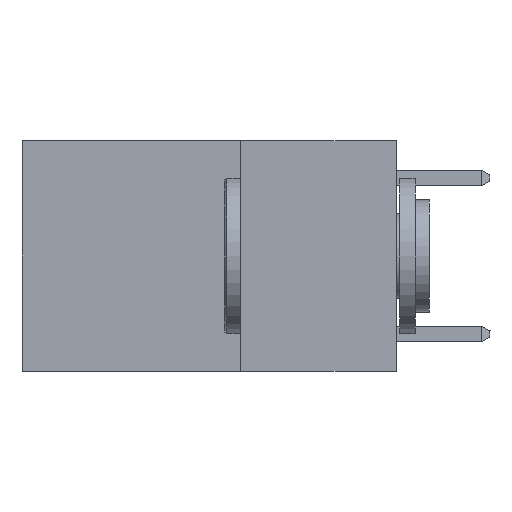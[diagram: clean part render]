
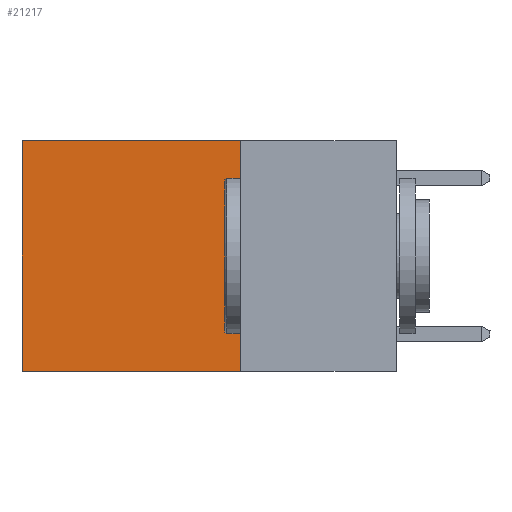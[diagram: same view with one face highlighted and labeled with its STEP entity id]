
A CAD part, left-side view. The second image highlights one B-rep face of the part: STEP entity #21217.
In plain terms, the highlighted planar face has unit normal (-1, 0, 0).
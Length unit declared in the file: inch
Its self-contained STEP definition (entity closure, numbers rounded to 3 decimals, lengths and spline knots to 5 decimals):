
#275 = CARTESIAN_POINT ( 'NONE',  ( 0.2625, 0.6, 0. ) ) ;
#626 = LINE ( 'NONE', #275, #7732 ) ;
#3592 = ORIENTED_EDGE ( 'NONE', *, *, #16844, .T. ) ;
#4262 = CARTESIAN_POINT ( 'NONE',  ( 0.2625, 0.25, -0.37 ) ) ;
#5651 = AXIS2_PLACEMENT_3D ( 'NONE', #19839, #7874, #24626 ) ;
#5946 = CARTESIAN_POINT ( 'NONE',  ( 0.2625, 0.25, 0. ) ) ;
#6872 = CARTESIAN_POINT ( 'NONE',  ( 0.2625, 0.25, -0.37 ) ) ;
#7732 = VECTOR ( 'NONE', #24258, 39.37008 ) ;
#7874 = DIRECTION ( 'NONE',  ( 1., 0., 0. ) ) ;
#11036 = FACE_OUTER_BOUND ( 'NONE', #11213, .T. ) ;
#11213 = EDGE_LOOP ( 'NONE', ( #16848, #19239, #18117, #3592 ) ) ;
#11928 = EDGE_CURVE ( 'NONE', #29138, #14892, #626, .T. ) ;
#12574 = PLANE ( 'NONE',  #5651 ) ;
#13385 = LINE ( 'NONE', #4262, #14127 ) ;
#13697 = EDGE_CURVE ( 'NONE', #24052, #15605, #14722, .T. ) ;
#14127 = VECTOR ( 'NONE', #21028, 39.37008 ) ;
#14722 = LINE ( 'NONE', #27965, #20397 ) ;
#14892 = VERTEX_POINT ( 'NONE', #18669 ) ;
#15488 = CARTESIAN_POINT ( 'NONE',  ( 0.2625, 0.6, 0. ) ) ;
#15605 = VERTEX_POINT ( 'NONE', #6872 ) ;
#15708 = CARTESIAN_POINT ( 'NONE',  ( 0.2625, 0.25, 0. ) ) ;
#16844 = EDGE_CURVE ( 'NONE', #24052, #29138, #19547, .T. ) ;
#16848 = ORIENTED_EDGE ( 'NONE', *, *, #11928, .T. ) ;
#18117 = ORIENTED_EDGE ( 'NONE', *, *, #13697, .F. ) ;
#18669 = CARTESIAN_POINT ( 'NONE',  ( 0.2625, 0.6, -0.37 ) ) ;
#19239 = ORIENTED_EDGE ( 'NONE', *, *, #20165, .F. ) ;
#19547 = LINE ( 'NONE', #5946, #30498 ) ;
#19839 = CARTESIAN_POINT ( 'NONE',  ( 0.2625, 0.25, 0. ) ) ;
#20165 = EDGE_CURVE ( 'NONE', #15605, #14892, #13385, .T. ) ;
#20397 = VECTOR ( 'NONE', #25717, 39.37008 ) ;
#21028 = DIRECTION ( 'NONE',  ( 0., 1., 0. ) ) ;
#21217 = ADVANCED_FACE ( 'NONE', ( #11036 ), #12574, .F. ) ;
#22849 = DIRECTION ( 'NONE',  ( 0., 1., 0. ) ) ;
#24052 = VERTEX_POINT ( 'NONE', #15708 ) ;
#24258 = DIRECTION ( 'NONE',  ( 0., 0., -1. ) ) ;
#24626 = DIRECTION ( 'NONE',  ( 0., 0., -1. ) ) ;
#25717 = DIRECTION ( 'NONE',  ( 0., 0., -1. ) ) ;
#27965 = CARTESIAN_POINT ( 'NONE',  ( 0.2625, 0.25, 0. ) ) ;
#29138 = VERTEX_POINT ( 'NONE', #15488 ) ;
#30498 = VECTOR ( 'NONE', #22849, 39.37008 ) ;
